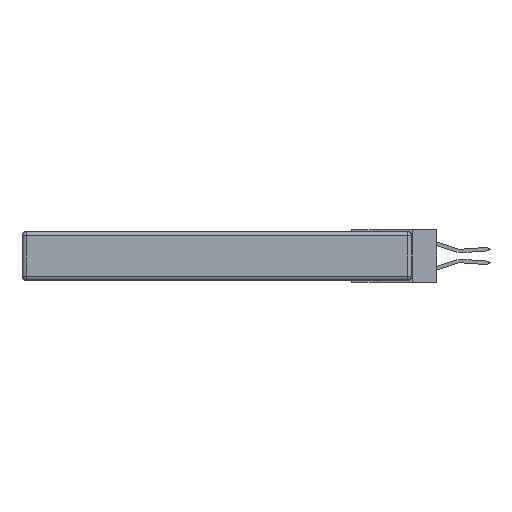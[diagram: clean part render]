
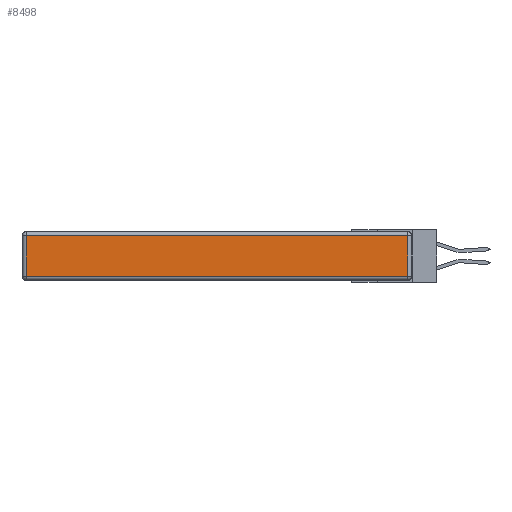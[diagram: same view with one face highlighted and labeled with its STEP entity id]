
A CAD part, left-side view. The second image highlights one B-rep face of the part: STEP entity #8498.
In plain terms, the highlighted planar face has unit normal (-1, 0, 0).
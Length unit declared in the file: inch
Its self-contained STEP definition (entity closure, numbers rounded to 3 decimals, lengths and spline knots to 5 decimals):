
#10 = LINE ( 'NONE', #18415, #21145 ) ;
#515 = LINE ( 'NONE', #11902, #4101 ) ;
#2166 = CARTESIAN_POINT ( 'NONE',  ( 0., 2.72, -0.313 ) ) ;
#3147 = ORIENTED_EDGE ( 'NONE', *, *, #19530, .T. ) ;
#3760 = ORIENTED_EDGE ( 'NONE', *, *, #4999, .T. ) ;
#4101 = VECTOR ( 'NONE', #14132, 39.37008 ) ;
#4194 = VERTEX_POINT ( 'NONE', #20133 ) ;
#4624 = VERTEX_POINT ( 'NONE', #18914 ) ;
#4999 = EDGE_CURVE ( 'NONE', #21569, #16520, #16243, .T. ) ;
#5054 = VECTOR ( 'NONE', #32383, 39.37008 ) ;
#7329 = ORIENTED_EDGE ( 'NONE', *, *, #8473, .T. ) ;
#7354 = EDGE_CURVE ( 'NONE', #4194, #4624, #515, .T. ) ;
#8473 = EDGE_CURVE ( 'NONE', #16520, #4194, #10, .T. ) ;
#8498 = ADVANCED_FACE ( 'NONE', ( #9220 ), #21418, .T. ) ;
#9220 = FACE_OUTER_BOUND ( 'NONE', #14600, .T. ) ;
#9485 = VECTOR ( 'NONE', #29654, 39.37008 ) ;
#10793 = DIRECTION ( 'NONE',  ( 0., -1., 0. ) ) ;
#11234 = DIRECTION ( 'NONE',  ( -1., 0., 0. ) ) ;
#11902 = CARTESIAN_POINT ( 'NONE',  ( 0., 0.03, -0.343 ) ) ;
#14132 = DIRECTION ( 'NONE',  ( 0., 0., 1. ) ) ;
#14600 = EDGE_LOOP ( 'NONE', ( #7329, #15349, #3147, #3760 ) ) ;
#15349 = ORIENTED_EDGE ( 'NONE', *, *, #7354, .T. ) ;
#16243 = LINE ( 'NONE', #24477, #9485 ) ;
#16520 = VERTEX_POINT ( 'NONE', #2166 ) ;
#17016 = CARTESIAN_POINT ( 'NONE',  ( 0., 2.75, -0.03 ) ) ;
#18204 = CARTESIAN_POINT ( 'NONE',  ( 0., 2.72, -0.03 ) ) ;
#18415 = CARTESIAN_POINT ( 'NONE',  ( 0., 0., -0.313 ) ) ;
#18914 = CARTESIAN_POINT ( 'NONE',  ( 0., 0.03, -0.03 ) ) ;
#19530 = EDGE_CURVE ( 'NONE', #4624, #21569, #27336, .T. ) ;
#20133 = CARTESIAN_POINT ( 'NONE',  ( 0., 0.03, -0.313 ) ) ;
#21145 = VECTOR ( 'NONE', #10793, 39.37008 ) ;
#21418 = PLANE ( 'NONE',  #21704 ) ;
#21569 = VERTEX_POINT ( 'NONE', #18204 ) ;
#21704 = AXIS2_PLACEMENT_3D ( 'NONE', #28694, #11234, #26315 ) ;
#24477 = CARTESIAN_POINT ( 'NONE',  ( 0., 2.72, -0.343 ) ) ;
#26315 = DIRECTION ( 'NONE',  ( 0., 0., 1. ) ) ;
#27336 = LINE ( 'NONE', #17016, #5054 ) ;
#28694 = CARTESIAN_POINT ( 'NONE',  ( 0., 0., -0.343 ) ) ;
#29654 = DIRECTION ( 'NONE',  ( 0., 0., -1. ) ) ;
#32383 = DIRECTION ( 'NONE',  ( 0., 1., 0. ) ) ;
